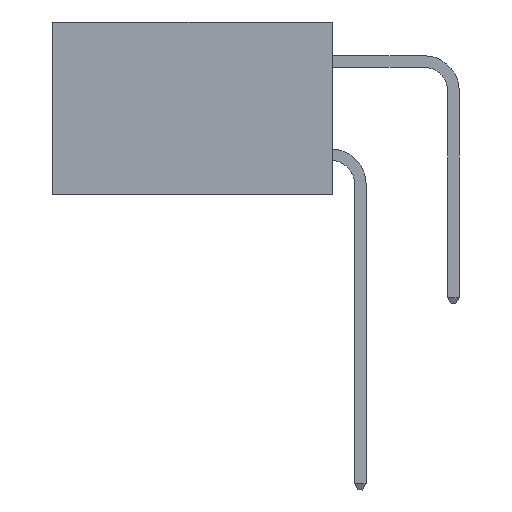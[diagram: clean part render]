
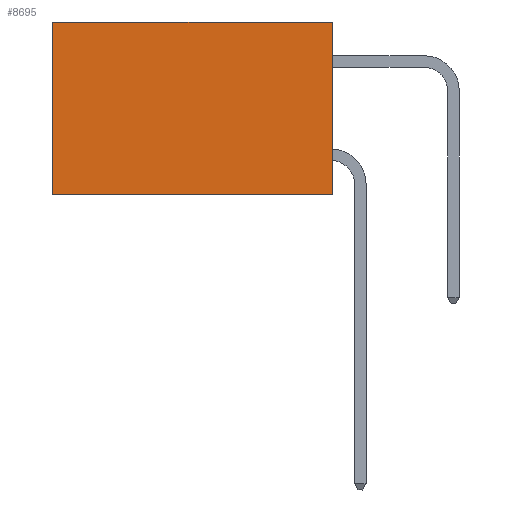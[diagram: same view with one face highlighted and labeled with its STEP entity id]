
A CAD part, left-side view. The second image highlights one B-rep face of the part: STEP entity #8695.
In plain terms, the highlighted planar face has unit normal (-1, 0, 0).
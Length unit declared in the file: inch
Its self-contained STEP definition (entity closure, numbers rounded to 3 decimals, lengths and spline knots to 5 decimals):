
#159 = CARTESIAN_POINT ( 'NONE',  ( 0.298, 0., -0.37 ) ) ;
#787 = PLANE ( 'NONE',  #5048 ) ;
#1414 = VERTEX_POINT ( 'NONE', #7826 ) ;
#1737 = VECTOR ( 'NONE', #2973, 39.37008 ) ;
#1865 = CARTESIAN_POINT ( 'NONE',  ( 0.298, 0.6, 0. ) ) ;
#2294 = CARTESIAN_POINT ( 'NONE',  ( 0.298, 0., 0. ) ) ;
#2681 = VERTEX_POINT ( 'NONE', #3126 ) ;
#2973 = DIRECTION ( 'NONE',  ( 0., 0., -1. ) ) ;
#3025 = LINE ( 'NONE', #10749, #11474 ) ;
#3126 = CARTESIAN_POINT ( 'NONE',  ( 0.298, 0., 0. ) ) ;
#3660 = DIRECTION ( 'NONE',  ( 0., 0., -1. ) ) ;
#4050 = LINE ( 'NONE', #159, #6826 ) ;
#4067 = DIRECTION ( 'NONE',  ( 1., 0., 0. ) ) ;
#4584 = ORIENTED_EDGE ( 'NONE', *, *, #6665, .F. ) ;
#4785 = EDGE_CURVE ( 'NONE', #2681, #12561, #7171, .T. ) ;
#5048 = AXIS2_PLACEMENT_3D ( 'NONE', #10089, #4067, #11155 ) ;
#5586 = ORIENTED_EDGE ( 'NONE', *, *, #9818, .T. ) ;
#6156 = EDGE_CURVE ( 'NONE', #1414, #11590, #4050, .T. ) ;
#6665 = EDGE_CURVE ( 'NONE', #2681, #1414, #3025, .T. ) ;
#6826 = VECTOR ( 'NONE', #10965, 39.37008 ) ;
#7171 = LINE ( 'NONE', #2294, #9447 ) ;
#7608 = LINE ( 'NONE', #1865, #1737 ) ;
#7826 = CARTESIAN_POINT ( 'NONE',  ( 0.298, 0., -0.37 ) ) ;
#8031 = CARTESIAN_POINT ( 'NONE',  ( 0.298, 0.6, -0.37 ) ) ;
#8136 = ORIENTED_EDGE ( 'NONE', *, *, #4785, .T. ) ;
#8176 = CARTESIAN_POINT ( 'NONE',  ( 0.298, 0.6, 0. ) ) ;
#8695 = ADVANCED_FACE ( 'NONE', ( #10271 ), #787, .F. ) ;
#9447 = VECTOR ( 'NONE', #9693, 39.37008 ) ;
#9693 = DIRECTION ( 'NONE',  ( 0., 1., 0. ) ) ;
#9818 = EDGE_CURVE ( 'NONE', #12561, #11590, #7608, .T. ) ;
#9880 = ORIENTED_EDGE ( 'NONE', *, *, #6156, .F. ) ;
#10089 = CARTESIAN_POINT ( 'NONE',  ( 0.298, 0., 0. ) ) ;
#10271 = FACE_OUTER_BOUND ( 'NONE', #11100, .T. ) ;
#10749 = CARTESIAN_POINT ( 'NONE',  ( 0.298, 0., 0. ) ) ;
#10965 = DIRECTION ( 'NONE',  ( 0., 1., 0. ) ) ;
#11100 = EDGE_LOOP ( 'NONE', ( #5586, #9880, #4584, #8136 ) ) ;
#11155 = DIRECTION ( 'NONE',  ( 0., 0., -1. ) ) ;
#11474 = VECTOR ( 'NONE', #3660, 39.37008 ) ;
#11590 = VERTEX_POINT ( 'NONE', #8031 ) ;
#12561 = VERTEX_POINT ( 'NONE', #8176 ) ;
